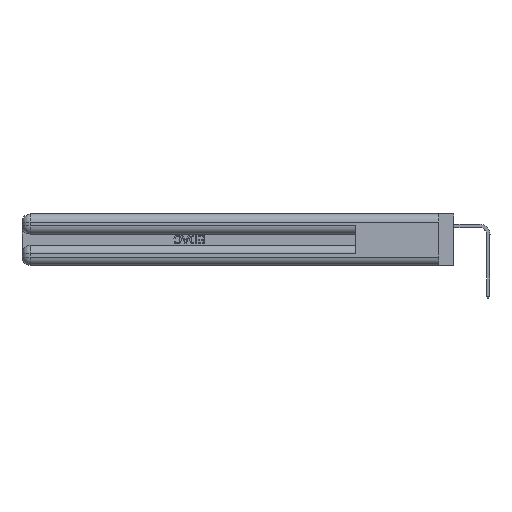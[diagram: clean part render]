
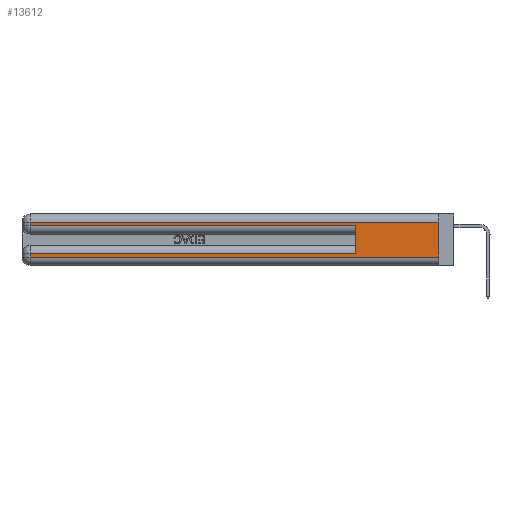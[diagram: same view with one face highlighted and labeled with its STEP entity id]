
A CAD part, left-side view. The second image highlights one B-rep face of the part: STEP entity #13612.
In plain terms, the highlighted planar face has unit normal (-1, 0, 0).
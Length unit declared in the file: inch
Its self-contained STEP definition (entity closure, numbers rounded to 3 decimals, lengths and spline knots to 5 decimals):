
#714 = CARTESIAN_POINT ( 'NONE',  ( 0., 0.6, 0.145 ) ) ;
#1938 = VERTEX_POINT ( 'NONE', #28034 ) ;
#3291 = DIRECTION ( 'NONE',  ( 0., 0., -1. ) ) ;
#3639 = ORIENTED_EDGE ( 'NONE', *, *, #15278, .T. ) ;
#3874 = VECTOR ( 'NONE', #37206, 39.37008 ) ;
#4537 = LINE ( 'NONE', #21964, #24816 ) ;
#5090 = CARTESIAN_POINT ( 'NONE',  ( 0., 2.94, 0.085 ) ) ;
#5729 = LINE ( 'NONE', #16252, #36867 ) ;
#6067 = DIRECTION ( 'NONE',  ( 0., 0., -1. ) ) ;
#7047 = FACE_OUTER_BOUND ( 'NONE', #30448, .T. ) ;
#7546 = VERTEX_POINT ( 'NONE', #24701 ) ;
#7704 = ORIENTED_EDGE ( 'NONE', *, *, #14660, .F. ) ;
#8214 = CARTESIAN_POINT ( 'NONE',  ( 0., 2.94, 0.06 ) ) ;
#9737 = VECTOR ( 'NONE', #17348, 39.37008 ) ;
#9785 = DIRECTION ( 'NONE',  ( 0., 0., -1. ) ) ;
#13174 = VECTOR ( 'NONE', #16003, 39.37008 ) ;
#13612 = ADVANCED_FACE ( 'NONE', ( #7047 ), #25944, .F. ) ;
#14274 = EDGE_CURVE ( 'NONE', #1938, #7546, #4537, .T. ) ;
#14605 = LINE ( 'NONE', #714, #3874 ) ;
#14660 = EDGE_CURVE ( 'NONE', #49504, #44667, #5729, .T. ) ;
#14811 = VERTEX_POINT ( 'NONE', #5090 ) ;
#15278 = EDGE_CURVE ( 'NONE', #14811, #31188, #48179, .T. ) ;
#15726 = AXIS2_PLACEMENT_3D ( 'NONE', #30099, #34170, #9785 ) ;
#16003 = DIRECTION ( 'NONE',  ( 0., 1., 0. ) ) ;
#16252 = CARTESIAN_POINT ( 'NONE',  ( 0., 0., 0.37 ) ) ;
#17348 = DIRECTION ( 'NONE',  ( 0., -1., 0. ) ) ;
#17381 = VERTEX_POINT ( 'NONE', #41687 ) ;
#19468 = VECTOR ( 'NONE', #6067, 39.37008 ) ;
#20535 = LINE ( 'NONE', #25358, #9737 ) ;
#21492 = ORIENTED_EDGE ( 'NONE', *, *, #38808, .T. ) ;
#21964 = CARTESIAN_POINT ( 'NONE',  ( 0., 0., 0.285 ) ) ;
#22396 = ORIENTED_EDGE ( 'NONE', *, *, #34386, .F. ) ;
#23575 = CARTESIAN_POINT ( 'NONE',  ( 0., 2.94, 0.31 ) ) ;
#23941 = DIRECTION ( 'NONE',  ( 0., 1., 0. ) ) ;
#24701 = CARTESIAN_POINT ( 'NONE',  ( 0., 0.6, 0.285 ) ) ;
#24816 = VECTOR ( 'NONE', #50337, 39.37008 ) ;
#25358 = CARTESIAN_POINT ( 'NONE',  ( 0., 0., 0.06 ) ) ;
#25944 = PLANE ( 'NONE',  #15726 ) ;
#26285 = CARTESIAN_POINT ( 'NONE',  ( 0., 2.94, 0.37 ) ) ;
#27567 = CARTESIAN_POINT ( 'NONE',  ( 0., 2.94, 0.37 ) ) ;
#27741 = ORIENTED_EDGE ( 'NONE', *, *, #48918, .T. ) ;
#28034 = CARTESIAN_POINT ( 'NONE',  ( 0., 2.94, 0.285 ) ) ;
#29593 = VECTOR ( 'NONE', #23941, 39.37008 ) ;
#29605 = ORIENTED_EDGE ( 'NONE', *, *, #31700, .T. ) ;
#30099 = CARTESIAN_POINT ( 'NONE',  ( 0., 0., 0.37 ) ) ;
#30448 = EDGE_LOOP ( 'NONE', ( #7704, #49712, #21492, #40652, #22396, #29605, #3639, #27741 ) ) ;
#30870 = LINE ( 'NONE', #44156, #29593 ) ;
#31188 = VERTEX_POINT ( 'NONE', #8214 ) ;
#31700 = EDGE_CURVE ( 'NONE', #17381, #14811, #30870, .T. ) ;
#34170 = DIRECTION ( 'NONE',  ( 1., 0., 0. ) ) ;
#34386 = EDGE_CURVE ( 'NONE', #17381, #7546, #14605, .T. ) ;
#34818 = LINE ( 'NONE', #44408, #13174 ) ;
#36867 = VECTOR ( 'NONE', #40587, 39.37008 ) ;
#37050 = CARTESIAN_POINT ( 'NONE',  ( 0., 0., 0.31 ) ) ;
#37206 = DIRECTION ( 'NONE',  ( 0., 0., 1. ) ) ;
#38492 = EDGE_CURVE ( 'NONE', #49504, #41408, #34818, .T. ) ;
#38702 = VECTOR ( 'NONE', #3291, 39.37008 ) ;
#38808 = EDGE_CURVE ( 'NONE', #41408, #1938, #39836, .T. ) ;
#39836 = LINE ( 'NONE', #26285, #19468 ) ;
#40587 = DIRECTION ( 'NONE',  ( 0., 0., -1. ) ) ;
#40652 = ORIENTED_EDGE ( 'NONE', *, *, #14274, .T. ) ;
#41408 = VERTEX_POINT ( 'NONE', #23575 ) ;
#41687 = CARTESIAN_POINT ( 'NONE',  ( 0., 0.6, 0.085 ) ) ;
#44156 = CARTESIAN_POINT ( 'NONE',  ( 0., 0., 0.085 ) ) ;
#44408 = CARTESIAN_POINT ( 'NONE',  ( 0., 0., 0.31 ) ) ;
#44667 = VERTEX_POINT ( 'NONE', #49673 ) ;
#48179 = LINE ( 'NONE', #27567, #38702 ) ;
#48918 = EDGE_CURVE ( 'NONE', #31188, #44667, #20535, .T. ) ;
#49504 = VERTEX_POINT ( 'NONE', #37050 ) ;
#49673 = CARTESIAN_POINT ( 'NONE',  ( 0., 0., 0.06 ) ) ;
#49712 = ORIENTED_EDGE ( 'NONE', *, *, #38492, .T. ) ;
#50337 = DIRECTION ( 'NONE',  ( 0., -1., 0. ) ) ;
